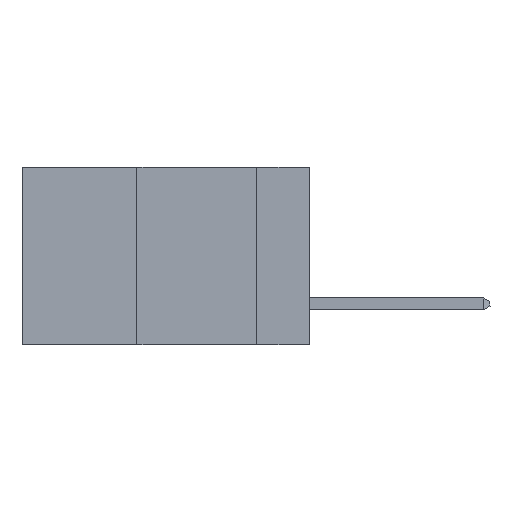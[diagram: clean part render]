
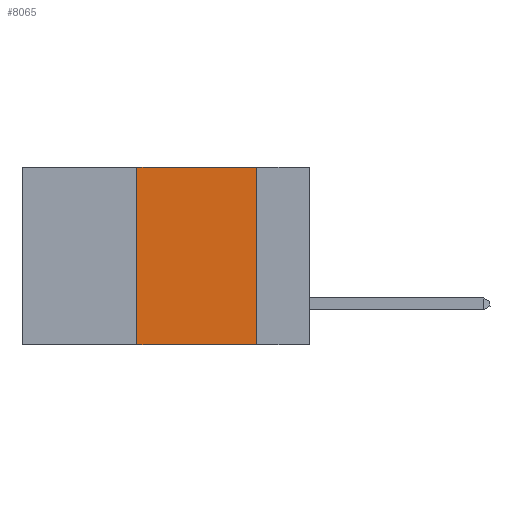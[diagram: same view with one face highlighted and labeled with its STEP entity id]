
A CAD part, left-side view. The second image highlights one B-rep face of the part: STEP entity #8065.
In plain terms, the highlighted planar face has unit normal (-1, 0, 0).
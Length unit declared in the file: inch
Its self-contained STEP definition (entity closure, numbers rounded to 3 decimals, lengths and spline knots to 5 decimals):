
#1259 = LINE ( 'NONE', #4397, #7055 ) ;
#1661 = CARTESIAN_POINT ( 'NONE',  ( 0., 0.6, 0. ) ) ;
#2530 = ORIENTED_EDGE ( 'NONE', *, *, #20935, .F. ) ;
#3328 = ORIENTED_EDGE ( 'NONE', *, *, #26592, .F. ) ;
#3469 = CARTESIAN_POINT ( 'NONE',  ( 0., 0.11, 0. ) ) ;
#3618 = PLANE ( 'NONE',  #5410 ) ;
#3984 = CARTESIAN_POINT ( 'NONE',  ( 0., 0.36, -0.37 ) ) ;
#4397 = CARTESIAN_POINT ( 'NONE',  ( 0., 0.6, -0.37 ) ) ;
#4609 = DIRECTION ( 'NONE',  ( 0., 0., 1. ) ) ;
#5410 = AXIS2_PLACEMENT_3D ( 'NONE', #18554, #7954, #22658 ) ;
#5898 = ORIENTED_EDGE ( 'NONE', *, *, #12095, .F. ) ;
#6912 = LINE ( 'NONE', #3469, #18241 ) ;
#7055 = VECTOR ( 'NONE', #19316, 39.37008 ) ;
#7755 = LINE ( 'NONE', #23621, #17769 ) ;
#7954 = DIRECTION ( 'NONE',  ( 1., 0., 0. ) ) ;
#8065 = ADVANCED_FACE ( 'NONE', ( #8336 ), #3618, .F. ) ;
#8336 = FACE_OUTER_BOUND ( 'NONE', #24440, .T. ) ;
#9933 = VERTEX_POINT ( 'NONE', #3984 ) ;
#11551 = VERTEX_POINT ( 'NONE', #15631 ) ;
#12095 = EDGE_CURVE ( 'NONE', #9933, #17509, #7755, .T. ) ;
#12466 = LINE ( 'NONE', #1661, #17438 ) ;
#15631 = CARTESIAN_POINT ( 'NONE',  ( 0., 0.11, -0.37 ) ) ;
#16324 = DIRECTION ( 'NONE',  ( 0., 0., -1. ) ) ;
#16741 = CARTESIAN_POINT ( 'NONE',  ( 0., 0.36, 0. ) ) ;
#17438 = VECTOR ( 'NONE', #18808, 39.37008 ) ;
#17509 = VERTEX_POINT ( 'NONE', #16741 ) ;
#17769 = VECTOR ( 'NONE', #4609, 39.37008 ) ;
#18241 = VECTOR ( 'NONE', #16324, 39.37008 ) ;
#18554 = CARTESIAN_POINT ( 'NONE',  ( 0., 0.6, 0. ) ) ;
#18808 = DIRECTION ( 'NONE',  ( 0., -1., 0. ) ) ;
#19316 = DIRECTION ( 'NONE',  ( 0., -1., 0. ) ) ;
#20935 = EDGE_CURVE ( 'NONE', #24999, #11551, #6912, .T. ) ;
#22658 = DIRECTION ( 'NONE',  ( 0., 0., -1. ) ) ;
#23621 = CARTESIAN_POINT ( 'NONE',  ( 0., 0.36, 0. ) ) ;
#23991 = CARTESIAN_POINT ( 'NONE',  ( 0., 0.11, 0. ) ) ;
#24057 = EDGE_CURVE ( 'NONE', #9933, #11551, #1259, .T. ) ;
#24440 = EDGE_LOOP ( 'NONE', ( #2530, #3328, #5898, #24955 ) ) ;
#24955 = ORIENTED_EDGE ( 'NONE', *, *, #24057, .T. ) ;
#24999 = VERTEX_POINT ( 'NONE', #23991 ) ;
#26592 = EDGE_CURVE ( 'NONE', #17509, #24999, #12466, .T. ) ;
